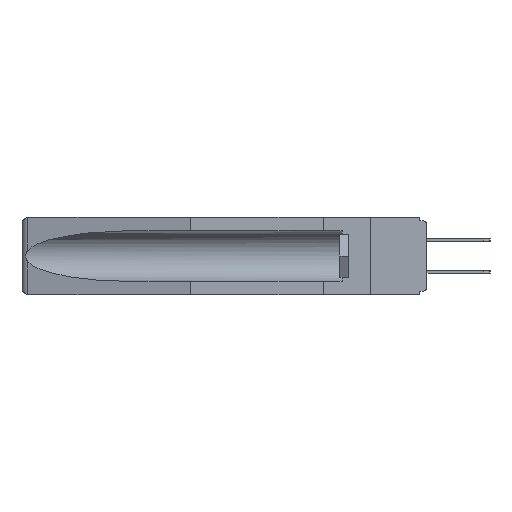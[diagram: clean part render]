
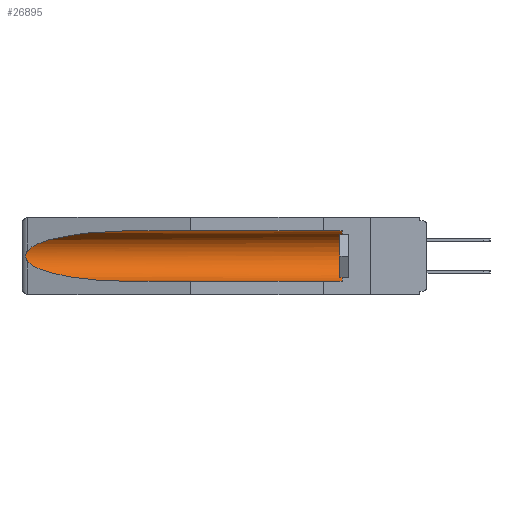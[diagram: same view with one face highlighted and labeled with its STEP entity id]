
A CAD part, left-side view. The second image highlights one B-rep face of the part: STEP entity #26895.
In plain terms, the highlighted cylindrical face has radius 2.857 mm (diameter 5.715 mm), a partial arc.
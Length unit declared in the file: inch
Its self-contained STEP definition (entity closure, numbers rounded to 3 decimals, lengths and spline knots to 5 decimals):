
#432 = CARTESIAN_POINT ( 'NONE',  ( 0.155, 1.07973, -0.284 ) ) ;
#1027 = CARTESIAN_POINT ( 'NONE',  ( 0.2675, 1.53308, -0.17534 ) ) ;
#2892 = VERTEX_POINT ( 'NONE', #432 ) ;
#3277 = CARTESIAN_POINT ( 'NONE',  ( 0.25451, 1.48313, -0.09465 ) ) ;
#3815 = CARTESIAN_POINT ( 'NONE',  ( 0.155, -0.30754, -0.059 ) ) ;
#3907 = LINE ( 'NONE', #3815, #12290 ) ;
#3909 = DIRECTION ( 'NONE',  ( 0., 1., 0. ) ) ;
#4092 = ORIENTED_EDGE ( 'NONE', *, *, #21480, .T. ) ;
#4383 = ORIENTED_EDGE ( 'NONE', *, *, #4899, .F. ) ;
#4490 = CARTESIAN_POINT ( 'NONE',  ( 0.26537, 1.52718, -0.19328 ) ) ;
#4899 = EDGE_CURVE ( 'NONE', #20665, #2892, #5134, .T. ) ;
#5134 = LINE ( 'NONE', #27454, #6794 ) ;
#5168 = ORIENTED_EDGE ( 'NONE', *, *, #26894, .T. ) ;
#5414 = CARTESIAN_POINT ( 'NONE',  ( 0.2673, 1.53269, -0.17917 ) ) ;
#5583 = CARTESIAN_POINT ( 'NONE',  ( 0.26597, 1.52961, -0.15275 ) ) ;
#6052 = CARTESIAN_POINT ( 'NONE',  ( 0.26537, 1.52718, -0.14972 ) ) ;
#6176 = FACE_OUTER_BOUND ( 'NONE', #7737, .T. ) ;
#6517 = CARTESIAN_POINT ( 'NONE',  ( 0.155, 0.126, -0.1715 ) ) ;
#6794 = VECTOR ( 'NONE', #21288, 39.37008 ) ;
#7156 = CARTESIAN_POINT ( 'NONE',  ( 0.26537, 1.52718, -0.19328 ) ) ;
#7172 = CARTESIAN_POINT ( 'NONE',  ( 0.21114, 1.30732, -0.284 ) ) ;
#7304 = EDGE_CURVE ( 'NONE', #20665, #10506, #14430, .T. ) ;
#7520 = AXIS2_PLACEMENT_3D ( 'NONE', #9588, #26562, #24767 ) ;
#7737 = EDGE_LOOP ( 'NONE', ( #5168, #4092, #24432, #4383, #24497, #26215 ) ) ;
#7754 = CARTESIAN_POINT ( 'NONE',  ( 0.26597, 1.5296, -0.19026 ) ) ;
#7975 = AXIS2_PLACEMENT_3D ( 'NONE', #6517, #23698, #25860 ) ;
#8227 =( BOUNDED_CURVE ( )  B_SPLINE_CURVE ( 3, ( #4490, #19505, #7172, #24451 ),
 .UNSPECIFIED., .F., .F. ) 
 B_SPLINE_CURVE_WITH_KNOTS ( ( 4, 4 ),
 ( 0.1948, 1.5708 ),
 .UNSPECIFIED. ) 
 CURVE ( )  GEOMETRIC_REPRESENTATION_ITEM ( )  RATIONAL_B_SPLINE_CURVE ( ( 1., 0.848, 0.848, 1. ) ) 
 REPRESENTATION_ITEM ( '' )  );
#9459 = B_SPLINE_CURVE_WITH_KNOTS ( 'NONE', 3,
 ( #22610, #5583, #22793, #27075, #14115, #1027, #5414, #20439, #7754, #9910 ),
 .UNSPECIFIED., .F., .F.,
 ( 4, 2, 2, 2, 4 ),
 ( 0., 0.00029, 0.00058, 0.00087, 0.00117 ),
 .UNSPECIFIED. ) ;
#9588 = CARTESIAN_POINT ( 'NONE',  ( 0.155, -0.30754, -0.1715 ) ) ;
#9910 = CARTESIAN_POINT ( 'NONE',  ( 0.26537, 1.52718, -0.19328 ) ) ;
#10506 = VERTEX_POINT ( 'NONE', #26616 ) ;
#12290 = VECTOR ( 'NONE', #3909, 39.37008 ) ;
#14115 = CARTESIAN_POINT ( 'NONE',  ( 0.2675, 1.53308, -0.16763 ) ) ;
#14126 = EDGE_CURVE ( 'NONE', #10506, #16199, #3907, .T. ) ;
#14204 = EDGE_CURVE ( 'NONE', #20528, #2892, #8227, .T. ) ;
#14430 = CIRCLE ( 'NONE', #7975, 0.1125 ) ;
#15265 =( BOUNDED_CURVE ( )  B_SPLINE_CURVE ( 3, ( #16026, #22539, #3277, #26918 ),
 .UNSPECIFIED., .F., .T. ) 
 B_SPLINE_CURVE_WITH_KNOTS ( ( 4, 4 ),
 ( 4.71239, 6.08839 ),
 .UNSPECIFIED. ) 
 CURVE ( )  GEOMETRIC_REPRESENTATION_ITEM ( )  RATIONAL_B_SPLINE_CURVE ( ( 1., 0.848, 0.848, 1. ) ) 
 REPRESENTATION_ITEM ( '' )  );
#15850 = VERTEX_POINT ( 'NONE', #6052 ) ;
#16026 = CARTESIAN_POINT ( 'NONE',  ( 0.155, 1.07973, -0.059 ) ) ;
#16199 = VERTEX_POINT ( 'NONE', #18125 ) ;
#18125 = CARTESIAN_POINT ( 'NONE',  ( 0.155, 1.07973, -0.059 ) ) ;
#19505 = CARTESIAN_POINT ( 'NONE',  ( 0.25451, 1.48313, -0.24835 ) ) ;
#20439 = CARTESIAN_POINT ( 'NONE',  ( 0.26655, 1.53094, -0.18657 ) ) ;
#20528 = VERTEX_POINT ( 'NONE', #7156 ) ;
#20665 = VERTEX_POINT ( 'NONE', #21101 ) ;
#21101 = CARTESIAN_POINT ( 'NONE',  ( 0.155, 0.126, -0.284 ) ) ;
#21288 = DIRECTION ( 'NONE',  ( 0., 1., 0. ) ) ;
#21480 = EDGE_CURVE ( 'NONE', #15850, #20528, #9459, .T. ) ;
#22539 = CARTESIAN_POINT ( 'NONE',  ( 0.21114, 1.30732, -0.059 ) ) ;
#22610 = CARTESIAN_POINT ( 'NONE',  ( 0.26537, 1.52718, -0.14972 ) ) ;
#22793 = CARTESIAN_POINT ( 'NONE',  ( 0.26654, 1.53092, -0.15636 ) ) ;
#23698 = DIRECTION ( 'NONE',  ( 0., -1., 0. ) ) ;
#24432 = ORIENTED_EDGE ( 'NONE', *, *, #14204, .T. ) ;
#24451 = CARTESIAN_POINT ( 'NONE',  ( 0.155, 1.07973, -0.284 ) ) ;
#24497 = ORIENTED_EDGE ( 'NONE', *, *, #7304, .T. ) ;
#24635 = CYLINDRICAL_SURFACE ( 'NONE', #7520, 0.1125 ) ;
#24767 = DIRECTION ( 'NONE',  ( 0., 0., 1. ) ) ;
#25860 = DIRECTION ( 'NONE',  ( 0., 0., 1. ) ) ;
#26215 = ORIENTED_EDGE ( 'NONE', *, *, #14126, .T. ) ;
#26562 = DIRECTION ( 'NONE',  ( 0., 1., 0. ) ) ;
#26616 = CARTESIAN_POINT ( 'NONE',  ( 0.155, 0.126, -0.059 ) ) ;
#26894 = EDGE_CURVE ( 'NONE', #16199, #15850, #15265, .T. ) ;
#26895 = ADVANCED_FACE ( 'NONE', ( #6176 ), #24635, .F. ) ;
#26918 = CARTESIAN_POINT ( 'NONE',  ( 0.26537, 1.52718, -0.14972 ) ) ;
#27075 = CARTESIAN_POINT ( 'NONE',  ( 0.2673, 1.5327, -0.16383 ) ) ;
#27454 = CARTESIAN_POINT ( 'NONE',  ( 0.155, -0.30754, -0.284 ) ) ;
